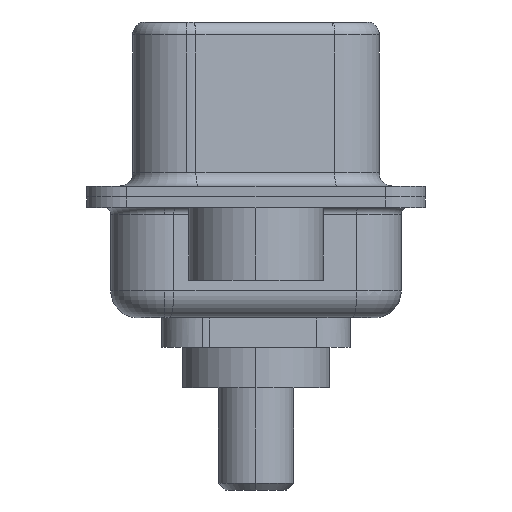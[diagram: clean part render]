
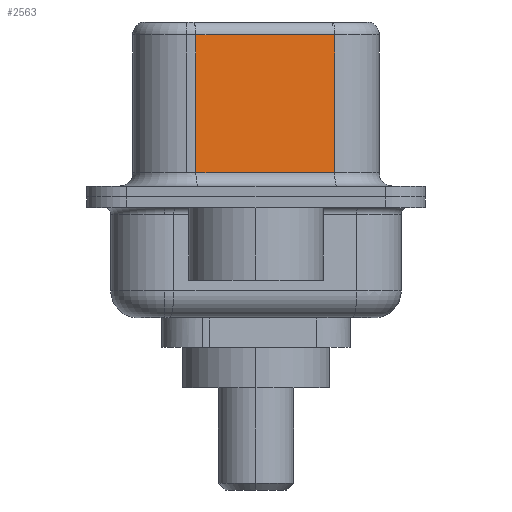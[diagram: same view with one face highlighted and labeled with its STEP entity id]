
A CAD part, left-side view. The second image highlights one B-rep face of the part: STEP entity #2563.
In plain terms, the highlighted planar face has unit normal (-0.985, -0.174, 0).
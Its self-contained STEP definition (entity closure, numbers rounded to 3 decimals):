
#17 = AXIS2_PLACEMENT_3D ( 'NONE', #149, #11729, #12050 ) ;
#149 = CARTESIAN_POINT ( 'NONE',  ( 4.58, -2.927, 6.52 ) ) ;
#559 = CARTESIAN_POINT ( 'NONE',  ( 4.58, -2.927, 6.02 ) ) ;
#673 = VECTOR ( 'NONE', #18114, 1000. ) ;
#919 = CARTESIAN_POINT ( 'NONE',  ( 4.58, -2.927, 0.9 ) ) ;
#2002 = DIRECTION ( 'NONE',  ( -0.174, 0.985, 0. ) ) ;
#2336 = DIRECTION ( 'NONE',  ( 0.174, -0.985, 0. ) ) ;
#2563 = ADVANCED_FACE ( 'NONE', ( #8886 ), #13110, .F. ) ;
#3432 = CARTESIAN_POINT ( 'NONE',  ( 4.58, -2.927, 6.52 ) ) ;
#3749 = EDGE_CURVE ( 'NONE', #9722, #13666, #18018, .T. ) ;
#4877 = DIRECTION ( 'NONE',  ( 0., 0., -1. ) ) ;
#6631 = CARTESIAN_POINT ( 'NONE',  ( 3.67, 2.233, 6.52 ) ) ;
#6775 = CARTESIAN_POINT ( 'NONE',  ( 3.67, 2.233, 0.9 ) ) ;
#7573 = VERTEX_POINT ( 'NONE', #14103 ) ;
#8211 = VECTOR ( 'NONE', #2002, 1000. ) ;
#8506 = LINE ( 'NONE', #3432, #673 ) ;
#8696 = EDGE_LOOP ( 'NONE', ( #13997, #17730, #13739, #10578 ) ) ;
#8842 = EDGE_CURVE ( 'NONE', #7573, #9722, #17138, .T. ) ;
#8886 = FACE_OUTER_BOUND ( 'NONE', #8696, .T. ) ;
#8972 = CARTESIAN_POINT ( 'NONE',  ( 3.67, 2.233, 6.02 ) ) ;
#9722 = VERTEX_POINT ( 'NONE', #8972 ) ;
#10578 = ORIENTED_EDGE ( 'NONE', *, *, #15331, .T. ) ;
#11400 = VERTEX_POINT ( 'NONE', #17177 ) ;
#11729 = DIRECTION ( 'NONE',  ( 0.985, 0.174, 0. ) ) ;
#12050 = DIRECTION ( 'NONE',  ( -0.174, 0.985, 0. ) ) ;
#12650 = LINE ( 'NONE', #919, #14690 ) ;
#13110 = PLANE ( 'NONE',  #17 ) ;
#13666 = VERTEX_POINT ( 'NONE', #6775 ) ;
#13739 = ORIENTED_EDGE ( 'NONE', *, *, #3749, .T. ) ;
#13997 = ORIENTED_EDGE ( 'NONE', *, *, #14471, .F. ) ;
#14103 = CARTESIAN_POINT ( 'NONE',  ( 4.58, -2.927, 6.02 ) ) ;
#14471 = EDGE_CURVE ( 'NONE', #7573, #11400, #8506, .T. ) ;
#14690 = VECTOR ( 'NONE', #2336, 1000. ) ;
#15331 = EDGE_CURVE ( 'NONE', #13666, #11400, #12650, .T. ) ;
#15974 = VECTOR ( 'NONE', #4877, 1000. ) ;
#17138 = LINE ( 'NONE', #559, #8211 ) ;
#17177 = CARTESIAN_POINT ( 'NONE',  ( 4.58, -2.927, 0.9 ) ) ;
#17730 = ORIENTED_EDGE ( 'NONE', *, *, #8842, .T. ) ;
#18018 = LINE ( 'NONE', #6631, #15974 ) ;
#18114 = DIRECTION ( 'NONE',  ( 0., 0., -1. ) ) ;
